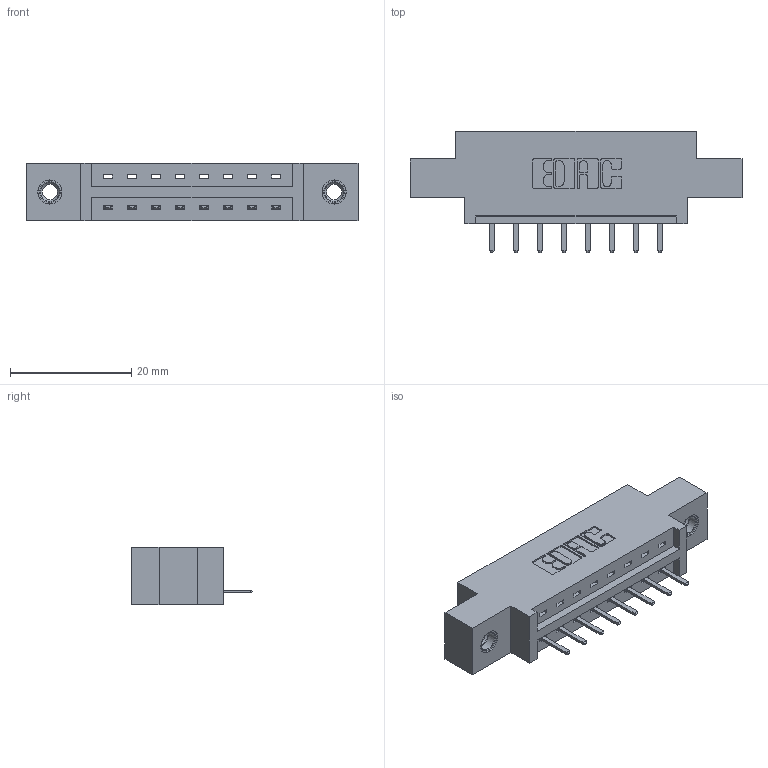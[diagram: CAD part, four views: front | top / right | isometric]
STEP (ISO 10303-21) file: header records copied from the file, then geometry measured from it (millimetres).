
FILE_DESCRIPTION (( 'STEP AP203' ), '1' );
FILE_NAME ('337-008-520-607.STEP', '2018-08-03T20:56:23', ( '' ), ( '' ), 'SwSTEP 2.0', 'SolidWorks 2016', '' );
FILE_SCHEMA (( 'CONFIG_CONTROL_DESIGN' ));
Length unit declared in the file: inch
Products named in the file (4): 337 Part_0.170 Offset - 0.156 Dia-TI; 345-292-001_345-293-120; 345-250-001_345-250-005-103; 337-008-520-607
Assembly tree (11 placements, depth 2):
  337-008-520-607
    337 Part_0.170 Offset - 0.156 Dia-TI
    345-292-001_345-293-120  x8
    345-250-001_345-250-005-103  x2
Bounding box: 54.71 x 20.02 x 9.4 mm (x, y, z)
Volume: 5106.8 mm3; surface area: 5143.1 mm2
Topology: 11 solids, 11 shells, 706 faces, 2027 edges, 1322 vertices
Faces by surface type: plane 490, cylinder 200, cone 12, torus 4
Entity records: 11776 total; most frequent: CARTESIAN_POINT 2041, ORIENTED_EDGE 1966, DIRECTION 1809, EDGE_CURVE 983, LINE 831, VECTOR 831, VERTEX_POINT 648, AXIS2_PLACEMENT_3D 489
